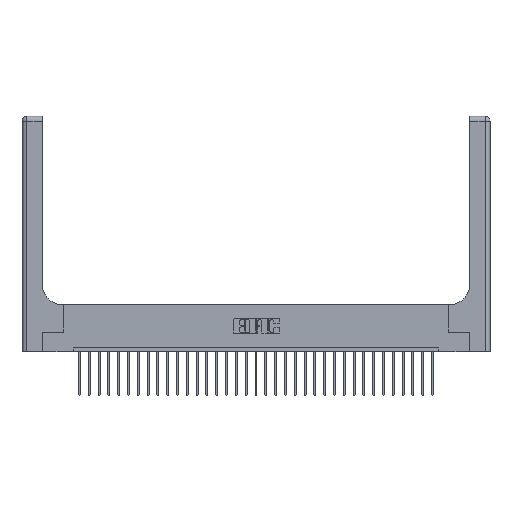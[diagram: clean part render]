
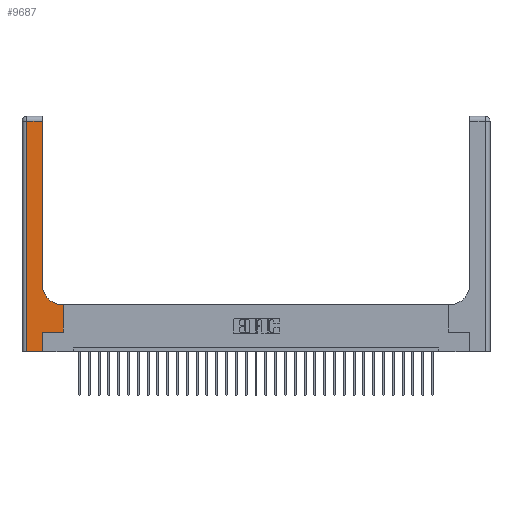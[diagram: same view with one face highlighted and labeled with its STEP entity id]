
A CAD part, top view. The second image highlights one B-rep face of the part: STEP entity #9687.
In plain terms, the highlighted planar face has unit normal (0, 0, 1).
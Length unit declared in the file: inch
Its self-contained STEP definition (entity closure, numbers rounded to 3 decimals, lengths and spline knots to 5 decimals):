
#369 = LINE ( 'NONE', #18148, #5294 ) ;
#1007 = DIRECTION ( 'NONE',  ( -1., 0., 0. ) ) ;
#1021 = VERTEX_POINT ( 'NONE', #10313 ) ;
#1729 = EDGE_LOOP ( 'NONE', ( #25735, #27932, #25468, #1835, #27340, #19300, #12691, #3030, #13342 ) ) ;
#1835 = ORIENTED_EDGE ( 'NONE', *, *, #8450, .T. ) ;
#2162 = CARTESIAN_POINT ( 'NONE',  ( 0.06, 2.94, 0.37 ) ) ;
#2375 = LINE ( 'NONE', #22054, #6204 ) ;
#2901 = VECTOR ( 'NONE', #15006, 39.37008 ) ;
#3030 = ORIENTED_EDGE ( 'NONE', *, *, #10800, .T. ) ;
#3129 = LINE ( 'NONE', #6449, #20456 ) ;
#3652 = VERTEX_POINT ( 'NONE', #9528 ) ;
#3789 = CIRCLE ( 'NONE', #17845, 0.25 ) ;
#4554 = VERTEX_POINT ( 'NONE', #25339 ) ;
#5261 = DIRECTION ( 'NONE',  ( -1., 0., 0. ) ) ;
#5294 = VECTOR ( 'NONE', #18058, 39.37008 ) ;
#5892 = LINE ( 'NONE', #27051, #21126 ) ;
#6204 = VECTOR ( 'NONE', #5261, 39.37008 ) ;
#6225 = VERTEX_POINT ( 'NONE', #2162 ) ;
#6449 = CARTESIAN_POINT ( 'NONE',  ( 0.265, 0.25, 0.37 ) ) ;
#8009 = DIRECTION ( 'NONE',  ( 0., 0., -1. ) ) ;
#8450 = EDGE_CURVE ( 'NONE', #16882, #4554, #369, .T. ) ;
#8759 = VERTEX_POINT ( 'NONE', #21893 ) ;
#8964 = EDGE_CURVE ( 'NONE', #1021, #18465, #19799, .T. ) ;
#9528 = CARTESIAN_POINT ( 'NONE',  ( 0.26, 2.94, 0.37 ) ) ;
#9687 = ADVANCED_FACE ( 'NONE', ( #22909 ), #18831, .F. ) ;
#10237 = EDGE_CURVE ( 'NONE', #4554, #27873, #5892, .T. ) ;
#10313 = CARTESIAN_POINT ( 'NONE',  ( 0.528, 0.25, 0.37 ) ) ;
#10357 = EDGE_CURVE ( 'NONE', #23811, #8759, #3789, .T. ) ;
#10800 = EDGE_CURVE ( 'NONE', #18465, #23811, #2375, .T. ) ;
#11213 = EDGE_CURVE ( 'NONE', #6225, #16882, #26987, .T. ) ;
#11923 = EDGE_CURVE ( 'NONE', #3652, #6225, #18966, .T. ) ;
#12006 = CARTESIAN_POINT ( 'NONE',  ( 0.528, 0.25, 0.37 ) ) ;
#12691 = ORIENTED_EDGE ( 'NONE', *, *, #8964, .T. ) ;
#13342 = ORIENTED_EDGE ( 'NONE', *, *, #10357, .T. ) ;
#14456 = CARTESIAN_POINT ( 'NONE',  ( 0.265, 0.25, 0.37 ) ) ;
#14560 = DIRECTION ( 'NONE',  ( -1., 0., 0. ) ) ;
#14839 = CARTESIAN_POINT ( 'NONE',  ( 0., 2.94, 0.37 ) ) ;
#14978 = CARTESIAN_POINT ( 'NONE',  ( 0.51, 0.85, 0.37 ) ) ;
#15006 = DIRECTION ( 'NONE',  ( 0., 1., 0. ) ) ;
#15858 = DIRECTION ( 'NONE',  ( 0., 1., 0. ) ) ;
#16545 = VECTOR ( 'NONE', #22192, 39.37008 ) ;
#16882 = VERTEX_POINT ( 'NONE', #26805 ) ;
#17156 = CARTESIAN_POINT ( 'NONE',  ( 0.26, 3., 0.37 ) ) ;
#17241 = VECTOR ( 'NONE', #14560, 39.37008 ) ;
#17845 = AXIS2_PLACEMENT_3D ( 'NONE', #14978, #8009, #25768 ) ;
#18058 = DIRECTION ( 'NONE',  ( 1., 0., 0. ) ) ;
#18148 = CARTESIAN_POINT ( 'NONE',  ( 0., 0., 0.37 ) ) ;
#18465 = VERTEX_POINT ( 'NONE', #21019 ) ;
#18831 = PLANE ( 'NONE',  #27367 ) ;
#18966 = LINE ( 'NONE', #14839, #17241 ) ;
#19300 = ORIENTED_EDGE ( 'NONE', *, *, #23812, .T. ) ;
#19799 = LINE ( 'NONE', #12006, #26435 ) ;
#20456 = VECTOR ( 'NONE', #26443, 39.37008 ) ;
#21019 = CARTESIAN_POINT ( 'NONE',  ( 0.528, 0.6, 0.37 ) ) ;
#21126 = VECTOR ( 'NONE', #15858, 39.37008 ) ;
#21467 = CARTESIAN_POINT ( 'NONE',  ( 0.51, 0.6, 0.37 ) ) ;
#21893 = CARTESIAN_POINT ( 'NONE',  ( 0.26, 0.85, 0.37 ) ) ;
#21957 = EDGE_CURVE ( 'NONE', #8759, #3652, #26497, .T. ) ;
#22054 = CARTESIAN_POINT ( 'NONE',  ( 0.26, 0.6, 0.37 ) ) ;
#22192 = DIRECTION ( 'NONE',  ( 0., -1., 0. ) ) ;
#22288 = CARTESIAN_POINT ( 'NONE',  ( 0.06, 3., 0.37 ) ) ;
#22909 = FACE_OUTER_BOUND ( 'NONE', #1729, .T. ) ;
#23211 = DIRECTION ( 'NONE',  ( 0., 0., -1. ) ) ;
#23811 = VERTEX_POINT ( 'NONE', #21467 ) ;
#23812 = EDGE_CURVE ( 'NONE', #27873, #1021, #3129, .T. ) ;
#25339 = CARTESIAN_POINT ( 'NONE',  ( 0.265, 0., 0.37 ) ) ;
#25468 = ORIENTED_EDGE ( 'NONE', *, *, #11213, .T. ) ;
#25650 = CARTESIAN_POINT ( 'NONE',  ( 0., 3., 0.37 ) ) ;
#25735 = ORIENTED_EDGE ( 'NONE', *, *, #21957, .T. ) ;
#25768 = DIRECTION ( 'NONE',  ( 1., 0., 0. ) ) ;
#26435 = VECTOR ( 'NONE', #27334, 39.37008 ) ;
#26443 = DIRECTION ( 'NONE',  ( 1., 0., 0. ) ) ;
#26497 = LINE ( 'NONE', #17156, #2901 ) ;
#26805 = CARTESIAN_POINT ( 'NONE',  ( 0.06, 0., 0.37 ) ) ;
#26987 = LINE ( 'NONE', #22288, #16545 ) ;
#27051 = CARTESIAN_POINT ( 'NONE',  ( 0.265, 0., 0.37 ) ) ;
#27334 = DIRECTION ( 'NONE',  ( 0., 1., 0. ) ) ;
#27340 = ORIENTED_EDGE ( 'NONE', *, *, #10237, .T. ) ;
#27367 = AXIS2_PLACEMENT_3D ( 'NONE', #25650, #23211, #1007 ) ;
#27873 = VERTEX_POINT ( 'NONE', #14456 ) ;
#27932 = ORIENTED_EDGE ( 'NONE', *, *, #11923, .T. ) ;
